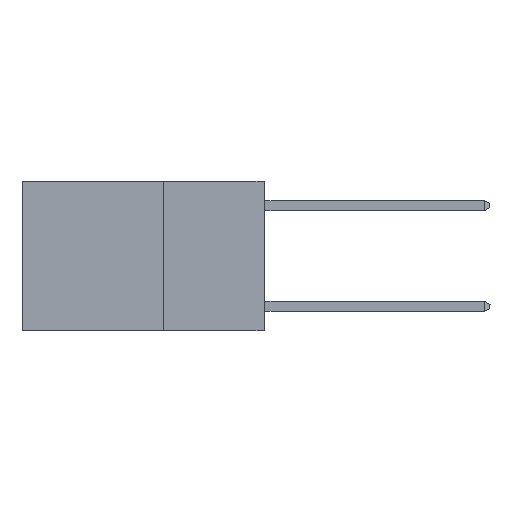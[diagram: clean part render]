
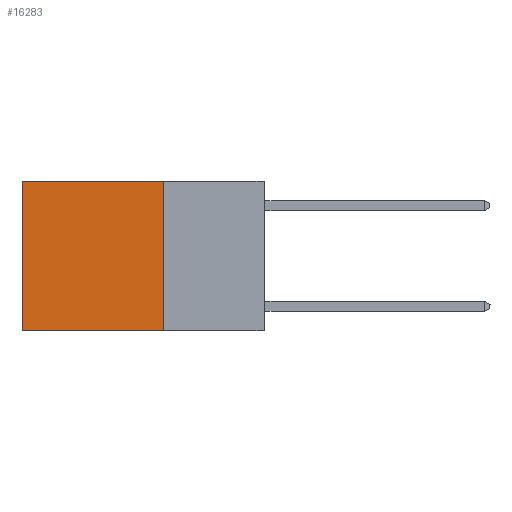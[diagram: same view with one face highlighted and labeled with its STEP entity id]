
A CAD part, left-side view. The second image highlights one B-rep face of the part: STEP entity #16283.
In plain terms, the highlighted planar face has unit normal (-1, 0, 0).
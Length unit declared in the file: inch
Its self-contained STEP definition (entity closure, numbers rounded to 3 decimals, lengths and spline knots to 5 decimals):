
#214 = VERTEX_POINT ( 'NONE', #8769 ) ;
#828 = DIRECTION ( 'NONE',  ( 0., 0., -1. ) ) ;
#2559 = VECTOR ( 'NONE', #828, 39.37008 ) ;
#2891 = VECTOR ( 'NONE', #15955, 39.37008 ) ;
#3547 = EDGE_CURVE ( 'NONE', #14704, #214, #7379, .T. ) ;
#5778 = DIRECTION ( 'NONE',  ( 0., 0., -1. ) ) ;
#5927 = CARTESIAN_POINT ( 'NONE',  ( 0.2625, 0.6, 0. ) ) ;
#6754 = FACE_OUTER_BOUND ( 'NONE', #20740, .T. ) ;
#7039 = VERTEX_POINT ( 'NONE', #17620 ) ;
#7213 = CARTESIAN_POINT ( 'NONE',  ( 0.2625, 0.25, 0. ) ) ;
#7379 = LINE ( 'NONE', #12605, #2891 ) ;
#7721 = EDGE_CURVE ( 'NONE', #14704, #7039, #12057, .T. ) ;
#7741 = ORIENTED_EDGE ( 'NONE', *, *, #14873, .T. ) ;
#7799 = ORIENTED_EDGE ( 'NONE', *, *, #20732, .F. ) ;
#8082 = ORIENTED_EDGE ( 'NONE', *, *, #7721, .F. ) ;
#8278 = VERTEX_POINT ( 'NONE', #20570 ) ;
#8769 = CARTESIAN_POINT ( 'NONE',  ( 0.2625, 0.6, 0. ) ) ;
#8850 = ORIENTED_EDGE ( 'NONE', *, *, #3547, .T. ) ;
#9746 = CARTESIAN_POINT ( 'NONE',  ( 0.2625, 0.25, -0.37 ) ) ;
#10030 = CARTESIAN_POINT ( 'NONE',  ( 0.2625, 0.25, 0. ) ) ;
#11735 = DIRECTION ( 'NONE',  ( 0., 0., -1. ) ) ;
#12057 = LINE ( 'NONE', #12563, #20870 ) ;
#12280 = VECTOR ( 'NONE', #19752, 39.37008 ) ;
#12563 = CARTESIAN_POINT ( 'NONE',  ( 0.2625, 0.25, 0. ) ) ;
#12605 = CARTESIAN_POINT ( 'NONE',  ( 0.2625, 0.25, 0. ) ) ;
#12805 = LINE ( 'NONE', #9746, #12280 ) ;
#14704 = VERTEX_POINT ( 'NONE', #7213 ) ;
#14873 = EDGE_CURVE ( 'NONE', #214, #8278, #16492, .T. ) ;
#15955 = DIRECTION ( 'NONE',  ( 0., 1., 0. ) ) ;
#16283 = ADVANCED_FACE ( 'NONE', ( #6754 ), #20017, .F. ) ;
#16492 = LINE ( 'NONE', #5927, #2559 ) ;
#17620 = CARTESIAN_POINT ( 'NONE',  ( 0.2625, 0.25, -0.37 ) ) ;
#18444 = AXIS2_PLACEMENT_3D ( 'NONE', #10030, #21644, #11735 ) ;
#19752 = DIRECTION ( 'NONE',  ( 0., 1., 0. ) ) ;
#20017 = PLANE ( 'NONE',  #18444 ) ;
#20570 = CARTESIAN_POINT ( 'NONE',  ( 0.2625, 0.6, -0.37 ) ) ;
#20732 = EDGE_CURVE ( 'NONE', #7039, #8278, #12805, .T. ) ;
#20740 = EDGE_LOOP ( 'NONE', ( #7741, #7799, #8082, #8850 ) ) ;
#20870 = VECTOR ( 'NONE', #5778, 39.37008 ) ;
#21644 = DIRECTION ( 'NONE',  ( 1., 0., 0. ) ) ;
